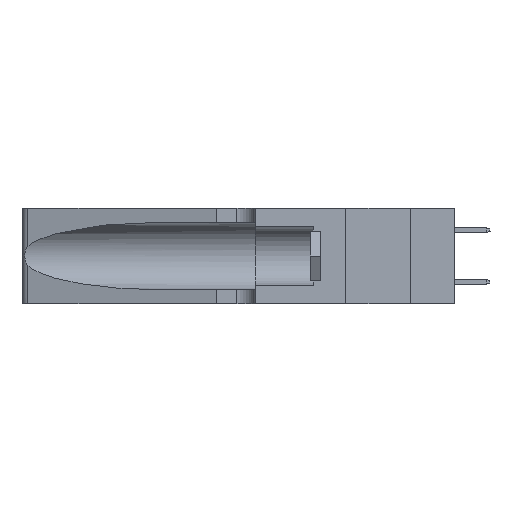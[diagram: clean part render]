
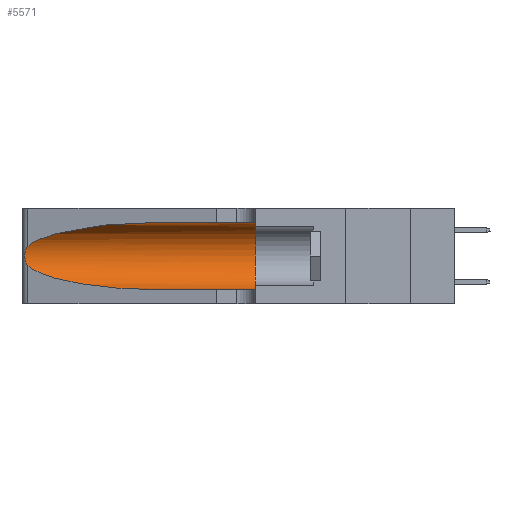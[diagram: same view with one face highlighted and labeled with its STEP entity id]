
A CAD part, left-side view. The second image highlights one B-rep face of the part: STEP entity #5571.
In plain terms, the highlighted cylindrical face has radius 3.308 mm (diameter 6.617 mm), a partial arc.
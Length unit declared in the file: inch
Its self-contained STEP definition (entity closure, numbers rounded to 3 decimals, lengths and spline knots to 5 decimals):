
#283 = CIRCLE ( 'NONE', #20930, 0.13025 ) ;
#1469 = CARTESIAN_POINT ( 'NONE',  ( 0.25487, 1.22718, 0.22369 ) ) ;
#1968 = LINE ( 'NONE', #17712, #2295 ) ;
#2008 = VERTEX_POINT ( 'NONE', #15115 ) ;
#2295 = VECTOR ( 'NONE', #9912, 39.37008 ) ;
#3325 = DIRECTION ( 'NONE',  ( 0., 1., 0. ) ) ;
#3725 = CARTESIAN_POINT ( 'NONE',  ( 0.25856, 1.23593, 0.16098 ) ) ;
#4390 = CARTESIAN_POINT ( 'NONE',  ( 0.25487, 1.22718, 0.22369 ) ) ;
#5047 = DIRECTION ( 'NONE',  ( 0., 0., -1. ) ) ;
#5075 = CARTESIAN_POINT ( 'NONE',  ( 0.1305, 0.72297, 0.05475 ) ) ;
#5331 = ORIENTED_EDGE ( 'NONE', *, *, #26045, .F. ) ;
#5571 = ADVANCED_FACE ( 'NONE', ( #25617 ), #12513, .F. ) ;
#5866 = VERTEX_POINT ( 'NONE', #24285 ) ;
#6227 = CARTESIAN_POINT ( 'NONE',  ( 0.26075, 1.23896, 0.178 ) ) ;
#6871 = CARTESIAN_POINT ( 'NONE',  ( 0.2373, 1.15595, 0.28018 ) ) ;
#7680 = B_SPLINE_CURVE_WITH_KNOTS ( 'NONE', 3,
 ( #23816, #26464, #10867, #20959, #8544, #21640, #8382, #6227, #16029, #3725, #11371, #31417, #21478, #18823 ),
 .UNSPECIFIED., .F., .F.,
 ( 4, 2, 2, 2, 2, 2, 4 ),
 ( 0., 0.00027, 0.00053, 0.00107, 0.0016, 0.00187, 0.00214 ),
 .UNSPECIFIED. ) ;
#8382 = CARTESIAN_POINT ( 'NONE',  ( 0.26075, 1.23896, 0.19203 ) ) ;
#8544 = CARTESIAN_POINT ( 'NONE',  ( 0.25854, 1.2359, 0.20912 ) ) ;
#8599 = ORIENTED_EDGE ( 'NONE', *, *, #17934, .T. ) ;
#8834 = ORIENTED_EDGE ( 'NONE', *, *, #28423, .T. ) ;
#9211 = CARTESIAN_POINT ( 'NONE',  ( 0.1305, 1.61858, 0.31525 ) ) ;
#9360 = CARTESIAN_POINT ( 'NONE',  ( 0.1305, 0.72297, 0.31525 ) ) ;
#9912 = DIRECTION ( 'NONE',  ( 0., -1., 0. ) ) ;
#10356 = VERTEX_POINT ( 'NONE', #1469 ) ;
#10867 = CARTESIAN_POINT ( 'NONE',  ( 0.25639, 1.23184, 0.21858 ) ) ;
#10972 = DIRECTION ( 'NONE',  ( 0., 0., 1. ) ) ;
#11371 = CARTESIAN_POINT ( 'NONE',  ( 0.25789, 1.23486, 0.15765 ) ) ;
#11383 = EDGE_CURVE ( 'NONE', #20585, #19191, #283, .T. ) ;
#12513 = CYLINDRICAL_SURFACE ( 'NONE', #15062, 0.13025 ) ;
#12671 = ORIENTED_EDGE ( 'NONE', *, *, #11383, .F. ) ;
#15062 = AXIS2_PLACEMENT_3D ( 'NONE', #30239, #22636, #5047 ) ;
#15115 = CARTESIAN_POINT ( 'NONE',  ( 0.1305, 0.72297, 0.31525 ) ) ;
#15141 = CARTESIAN_POINT ( 'NONE',  ( 0.1305, 0.35, 0.31525 ) ) ;
#15967 = ORIENTED_EDGE ( 'NONE', *, *, #28258, .T. ) ;
#16029 = CARTESIAN_POINT ( 'NONE',  ( 0.26017, 1.23833, 0.17102 ) ) ;
#16219 = EDGE_LOOP ( 'NONE', ( #8834, #8599, #15967, #30970, #12671, #5331 ) ) ;
#17712 = CARTESIAN_POINT ( 'NONE',  ( 0.1305, 1.61858, 0.05475 ) ) ;
#17934 = EDGE_CURVE ( 'NONE', #10356, #5866, #7680, .T. ) ;
#18667 = CARTESIAN_POINT ( 'NONE',  ( 0.1305, 0.72297, 0.05475 ) ) ;
#18823 = CARTESIAN_POINT ( 'NONE',  ( 0.25487, 1.22718, 0.14631 ) ) ;
#18991 = LINE ( 'NONE', #9211, #21481 ) ;
#19191 = VERTEX_POINT ( 'NONE', #29830 ) ;
#19475 = CARTESIAN_POINT ( 'NONE',  ( 0.18966, 0.96281, 0.31525 ) ) ;
#19625 =( BOUNDED_CURVE ( )  B_SPLINE_CURVE ( 3, ( #30589, #22997, #20654, #5075 ),
 .UNSPECIFIED., .F., .T. ) 
 B_SPLINE_CURVE_WITH_KNOTS ( ( 4, 4 ),
 ( 3.44316, 4.71239 ),
 .UNSPECIFIED. ) 
 CURVE ( )  GEOMETRIC_REPRESENTATION_ITEM ( )  RATIONAL_B_SPLINE_CURVE ( ( 1., 0.87, 0.87, 1. ) ) 
 REPRESENTATION_ITEM ( '' )  );
#20585 = VERTEX_POINT ( 'NONE', #15141 ) ;
#20654 = CARTESIAN_POINT ( 'NONE',  ( 0.18966, 0.96281, 0.05475 ) ) ;
#20930 = AXIS2_PLACEMENT_3D ( 'NONE', #26069, #3325, #10972 ) ;
#20959 = CARTESIAN_POINT ( 'NONE',  ( 0.25787, 1.23484, 0.2124 ) ) ;
#21478 = CARTESIAN_POINT ( 'NONE',  ( 0.25555, 1.22993, 0.14849 ) ) ;
#21481 = VECTOR ( 'NONE', #27284, 39.37008 ) ;
#21640 = CARTESIAN_POINT ( 'NONE',  ( 0.26018, 1.23835, 0.19895 ) ) ;
#22636 = DIRECTION ( 'NONE',  ( 0., -1., 0. ) ) ;
#22709 = EDGE_CURVE ( 'NONE', #31003, #19191, #1968, .T. ) ;
#22997 = CARTESIAN_POINT ( 'NONE',  ( 0.2373, 1.15595, 0.08982 ) ) ;
#23009 =( BOUNDED_CURVE ( )  B_SPLINE_CURVE ( 3, ( #9360, #19475, #6871, #4390 ),
 .UNSPECIFIED., .F., .T. ) 
 B_SPLINE_CURVE_WITH_KNOTS ( ( 4, 4 ),
 ( 1.5708, 2.84003 ),
 .UNSPECIFIED. ) 
 CURVE ( )  GEOMETRIC_REPRESENTATION_ITEM ( )  RATIONAL_B_SPLINE_CURVE ( ( 1., 0.87, 0.87, 1. ) ) 
 REPRESENTATION_ITEM ( '' )  );
#23816 = CARTESIAN_POINT ( 'NONE',  ( 0.25487, 1.22718, 0.22369 ) ) ;
#24285 = CARTESIAN_POINT ( 'NONE',  ( 0.25487, 1.22718, 0.14631 ) ) ;
#25617 = FACE_OUTER_BOUND ( 'NONE', #16219, .T. ) ;
#26045 = EDGE_CURVE ( 'NONE', #2008, #20585, #18991, .T. ) ;
#26069 = CARTESIAN_POINT ( 'NONE',  ( 0.1305, 0.35, 0.185 ) ) ;
#26464 = CARTESIAN_POINT ( 'NONE',  ( 0.25555, 1.22994, 0.2215 ) ) ;
#27284 = DIRECTION ( 'NONE',  ( 0., -1., 0. ) ) ;
#28258 = EDGE_CURVE ( 'NONE', #5866, #31003, #19625, .T. ) ;
#28423 = EDGE_CURVE ( 'NONE', #2008, #10356, #23009, .T. ) ;
#29830 = CARTESIAN_POINT ( 'NONE',  ( 0.1305, 0.35, 0.05475 ) ) ;
#30239 = CARTESIAN_POINT ( 'NONE',  ( 0.1305, 1.61858, 0.185 ) ) ;
#30589 = CARTESIAN_POINT ( 'NONE',  ( 0.25487, 1.22718, 0.14631 ) ) ;
#30970 = ORIENTED_EDGE ( 'NONE', *, *, #22709, .T. ) ;
#31003 = VERTEX_POINT ( 'NONE', #18667 ) ;
#31417 = CARTESIAN_POINT ( 'NONE',  ( 0.25639, 1.23186, 0.15144 ) ) ;
